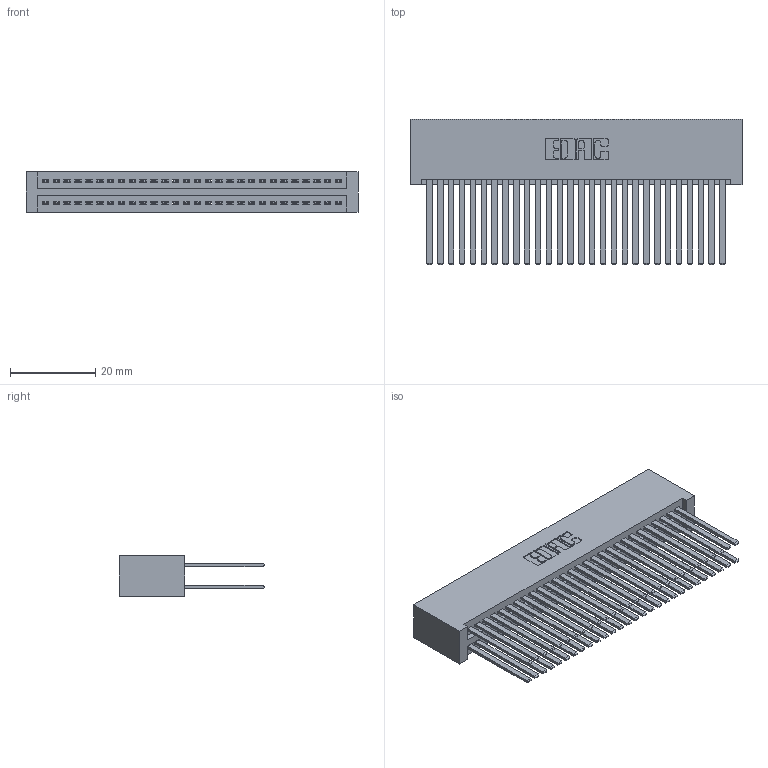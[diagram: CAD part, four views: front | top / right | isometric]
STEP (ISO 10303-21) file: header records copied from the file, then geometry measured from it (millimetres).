
FILE_DESCRIPTION (( 'STEP AP203' ), '1' );
FILE_NAME ('395-056-544-201.STEP', '2018-11-22T05:06:28', ( '' ), ( '' ), 'SwSTEP 2.0', 'SolidWorks 2016', '' );
FILE_SCHEMA (( 'CONFIG_CONTROL_DESIGN' ));
Length unit declared in the file: inch
Products named in the file (3): 345 Part_No Mounting Lugs; 345-292-001_345-293-144; 395-056-544-201
Assembly tree (57 placements, depth 2):
  395-056-544-201
    345 Part_No Mounting Lugs
    345-292-001_345-293-144  x56
Bounding box: 77.72 x 33.96 x 9.4 mm (x, y, z)
Volume: 8821.2 mm3; surface area: 15372.1 mm2
Topology: 57 solids, 57 shells, 2582 faces, 7653 edges, 5026 vertices
Faces by surface type: plane 1700, cylinder 882
Entity records: 23393 total; most frequent: CARTESIAN_POINT 3932, ORIENTED_EDGE 3866, DIRECTION 3477, EDGE_CURVE 1933, VECTOR 1701, LINE 1701, VERTEX_POINT 1286, AXIS2_PLACEMENT_3D 888
